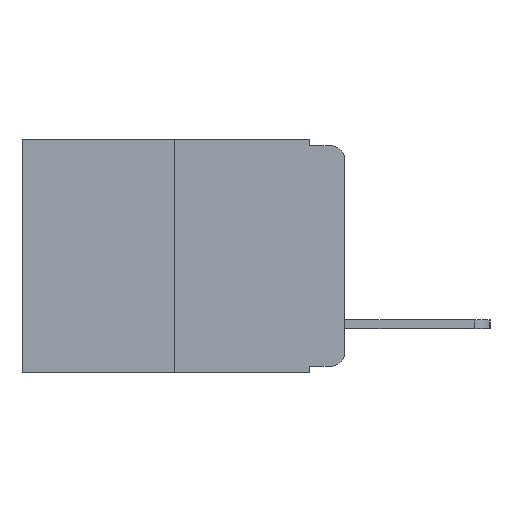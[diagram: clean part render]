
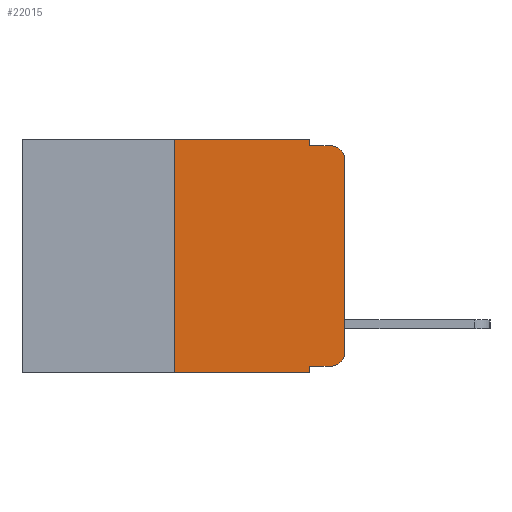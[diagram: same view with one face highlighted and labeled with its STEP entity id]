
A CAD part, left-side view. The second image highlights one B-rep face of the part: STEP entity #22015.
In plain terms, the highlighted planar face has unit normal (-1, 0, 0).
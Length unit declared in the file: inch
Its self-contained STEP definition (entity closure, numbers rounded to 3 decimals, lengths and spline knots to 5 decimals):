
#48 = CARTESIAN_POINT ( 'NONE',  ( 0., 0.051, -0.343 ) ) ;
#192 = VERTEX_POINT ( 'NONE', #20119 ) ;
#814 = ORIENTED_EDGE ( 'NONE', *, *, #3925, .F. ) ;
#860 = CARTESIAN_POINT ( 'NONE',  ( 0., 0.051, 0. ) ) ;
#909 = DIRECTION ( 'NONE',  ( 0., 0., -1. ) ) ;
#937 = CARTESIAN_POINT ( 'NONE',  ( 0., 0.25, -0.343 ) ) ;
#999 = AXIS2_PLACEMENT_3D ( 'NONE', #2003, #21780, #11248 ) ;
#1274 = VERTEX_POINT ( 'NONE', #6944 ) ;
#1380 = ORIENTED_EDGE ( 'NONE', *, *, #23286, .F. ) ;
#1517 = VERTEX_POINT ( 'NONE', #6735 ) ;
#1578 = VECTOR ( 'NONE', #17044, 39.37008 ) ;
#1843 = AXIS2_PLACEMENT_3D ( 'NONE', #9755, #22096, #11571 ) ;
#2002 = LINE ( 'NONE', #860, #6360 ) ;
#2003 = CARTESIAN_POINT ( 'NONE',  ( 0., 0.473, 0. ) ) ;
#2012 = VERTEX_POINT ( 'NONE', #2566 ) ;
#2440 = VERTEX_POINT ( 'NONE', #937 ) ;
#2468 = EDGE_CURVE ( 'NONE', #20102, #14977, #2002, .T. ) ;
#2566 = CARTESIAN_POINT ( 'NONE',  ( 0., 0., -0.03 ) ) ;
#3359 = VECTOR ( 'NONE', #20147, 39.37008 ) ;
#3925 = EDGE_CURVE ( 'NONE', #192, #20102, #19718, .T. ) ;
#4029 = ORIENTED_EDGE ( 'NONE', *, *, #2468, .F. ) ;
#4179 = DIRECTION ( 'NONE',  ( 0., -1., 0. ) ) ;
#4616 = DIRECTION ( 'NONE',  ( 0., -1., 0. ) ) ;
#4775 = EDGE_LOOP ( 'NONE', ( #11146, #14511, #6591, #4029, #814, #1380, #11167, #6900, #21103, #21631 ) ) ;
#5063 = AXIS2_PLACEMENT_3D ( 'NONE', #6217, #18742, #8079 ) ;
#5190 = VECTOR ( 'NONE', #12432, 39.37008 ) ;
#5452 = VECTOR ( 'NONE', #4616, 39.37008 ) ;
#5731 = PLANE ( 'NONE',  #999 ) ;
#6217 = CARTESIAN_POINT ( 'NONE',  ( 0., 0.02, -0.313 ) ) ;
#6360 = VECTOR ( 'NONE', #909, 39.37008 ) ;
#6591 = ORIENTED_EDGE ( 'NONE', *, *, #9891, .F. ) ;
#6735 = CARTESIAN_POINT ( 'NONE',  ( 0., 0., -0.313 ) ) ;
#6900 = ORIENTED_EDGE ( 'NONE', *, *, #21000, .F. ) ;
#6944 = CARTESIAN_POINT ( 'NONE',  ( 0., 0.02, -0.01 ) ) ;
#6970 = VECTOR ( 'NONE', #11980, 39.37008 ) ;
#7668 = VERTEX_POINT ( 'NONE', #15743 ) ;
#8079 = DIRECTION ( 'NONE',  ( 0., 0., -1. ) ) ;
#8193 = CIRCLE ( 'NONE', #5063, 0.02 ) ;
#8888 = LINE ( 'NONE', #18535, #22453 ) ;
#9755 = CARTESIAN_POINT ( 'NONE',  ( 0., 0.02, -0.03 ) ) ;
#9876 = CARTESIAN_POINT ( 'NONE',  ( 0., 0.051, 0. ) ) ;
#9891 = EDGE_CURVE ( 'NONE', #14977, #1274, #8888, .T. ) ;
#11146 = ORIENTED_EDGE ( 'NONE', *, *, #19368, .T. ) ;
#11167 = ORIENTED_EDGE ( 'NONE', *, *, #13820, .T. ) ;
#11248 = DIRECTION ( 'NONE',  ( 0., 0., -1. ) ) ;
#11571 = DIRECTION ( 'NONE',  ( 0., 0., -1. ) ) ;
#11826 = LINE ( 'NONE', #22501, #6970 ) ;
#11980 = DIRECTION ( 'NONE',  ( 0., 0., 1. ) ) ;
#12432 = DIRECTION ( 'NONE',  ( 0., 0., -1. ) ) ;
#12755 = EDGE_CURVE ( 'NONE', #7668, #1517, #8193, .T. ) ;
#12976 = CARTESIAN_POINT ( 'NONE',  ( 0., 0.051, -0.01 ) ) ;
#13582 = CARTESIAN_POINT ( 'NONE',  ( 0., 0.051, -0.333 ) ) ;
#13820 = EDGE_CURVE ( 'NONE', #2440, #14946, #22384, .T. ) ;
#13944 = EDGE_CURVE ( 'NONE', #15820, #7668, #15008, .T. ) ;
#14511 = ORIENTED_EDGE ( 'NONE', *, *, #17055, .T. ) ;
#14946 = VERTEX_POINT ( 'NONE', #48 ) ;
#14977 = VERTEX_POINT ( 'NONE', #12976 ) ;
#15008 = LINE ( 'NONE', #13582, #1578 ) ;
#15063 = FACE_OUTER_BOUND ( 'NONE', #4775, .T. ) ;
#15624 = CARTESIAN_POINT ( 'NONE',  ( 0., 0.473, 0. ) ) ;
#15743 = CARTESIAN_POINT ( 'NONE',  ( 0., 0.02, -0.333 ) ) ;
#15820 = VERTEX_POINT ( 'NONE', #17277 ) ;
#16737 = CARTESIAN_POINT ( 'NONE',  ( 0., 0.473, -0.343 ) ) ;
#17044 = DIRECTION ( 'NONE',  ( 0., -1., 0. ) ) ;
#17055 = EDGE_CURVE ( 'NONE', #2012, #1274, #17091, .T. ) ;
#17091 = CIRCLE ( 'NONE', #1843, 0.02 ) ;
#17277 = CARTESIAN_POINT ( 'NONE',  ( 0., 0.051, -0.333 ) ) ;
#17298 = DIRECTION ( 'NONE',  ( 0., 0., 1. ) ) ;
#17664 = VECTOR ( 'NONE', #17298, 39.37008 ) ;
#18535 = CARTESIAN_POINT ( 'NONE',  ( 0., 0.051, -0.01 ) ) ;
#18742 = DIRECTION ( 'NONE',  ( -1., 0., 0. ) ) ;
#18934 = LINE ( 'NONE', #22919, #5190 ) ;
#19368 = EDGE_CURVE ( 'NONE', #1517, #2012, #11826, .T. ) ;
#19718 = LINE ( 'NONE', #15624, #5452 ) ;
#20102 = VERTEX_POINT ( 'NONE', #9876 ) ;
#20119 = CARTESIAN_POINT ( 'NONE',  ( 0., 0.25, 0. ) ) ;
#20147 = DIRECTION ( 'NONE',  ( 0., -1., 0. ) ) ;
#21000 = EDGE_CURVE ( 'NONE', #15820, #14946, #18934, .T. ) ;
#21103 = ORIENTED_EDGE ( 'NONE', *, *, #13944, .T. ) ;
#21631 = ORIENTED_EDGE ( 'NONE', *, *, #12755, .T. ) ;
#21780 = DIRECTION ( 'NONE',  ( 1., 0., 0. ) ) ;
#22015 = ADVANCED_FACE ( 'NONE', ( #15063 ), #5731, .F. ) ;
#22096 = DIRECTION ( 'NONE',  ( -1., 0., 0. ) ) ;
#22384 = LINE ( 'NONE', #16737, #3359 ) ;
#22453 = VECTOR ( 'NONE', #4179, 39.37008 ) ;
#22501 = CARTESIAN_POINT ( 'NONE',  ( 0., 0., 0. ) ) ;
#22552 = CARTESIAN_POINT ( 'NONE',  ( 0., 0.25, 0. ) ) ;
#22827 = LINE ( 'NONE', #22552, #17664 ) ;
#22919 = CARTESIAN_POINT ( 'NONE',  ( 0., 0.051, 0. ) ) ;
#23286 = EDGE_CURVE ( 'NONE', #2440, #192, #22827, .T. ) ;
